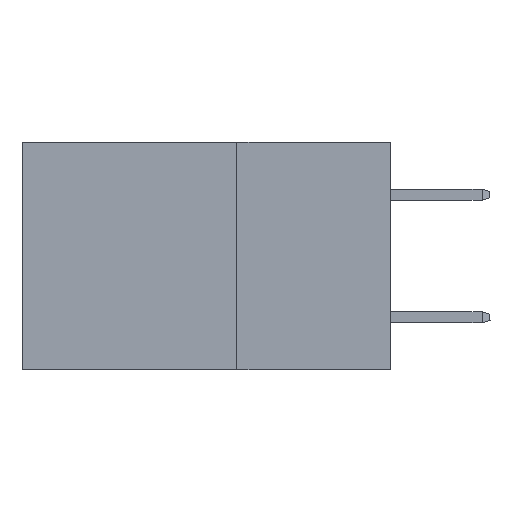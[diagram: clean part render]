
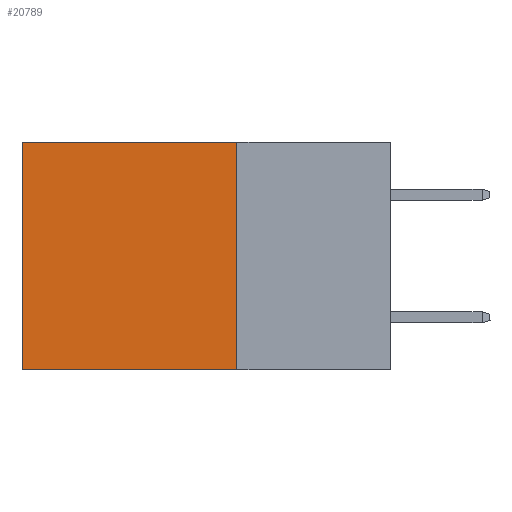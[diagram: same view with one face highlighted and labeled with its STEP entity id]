
A CAD part, left-side view. The second image highlights one B-rep face of the part: STEP entity #20789.
In plain terms, the highlighted planar face has unit normal (-1, 0, 0).
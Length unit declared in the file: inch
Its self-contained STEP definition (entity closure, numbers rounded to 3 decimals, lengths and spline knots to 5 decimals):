
#179 = DIRECTION ( 'NONE',  ( 0., 0., -1. ) ) ;
#887 = CARTESIAN_POINT ( 'NONE',  ( 0.2875, 0.25, 0. ) ) ;
#1106 = ORIENTED_EDGE ( 'NONE', *, *, #20926, .F. ) ;
#1913 = CARTESIAN_POINT ( 'NONE',  ( 0.2875, 0.6, 0. ) ) ;
#2788 = VERTEX_POINT ( 'NONE', #16098 ) ;
#2804 = CARTESIAN_POINT ( 'NONE',  ( 0.2875, 0.6, -0.37 ) ) ;
#3386 = VECTOR ( 'NONE', #23028, 39.37008 ) ;
#3429 = DIRECTION ( 'NONE',  ( 1., 0., 0. ) ) ;
#5271 = LINE ( 'NONE', #19650, #3386 ) ;
#5788 = CARTESIAN_POINT ( 'NONE',  ( 0.2875, 0.6, 0. ) ) ;
#6047 = DIRECTION ( 'NONE',  ( 0., 0., -1. ) ) ;
#6865 = LINE ( 'NONE', #1913, #8237 ) ;
#7371 = CARTESIAN_POINT ( 'NONE',  ( 0.2875, 0.25, 0. ) ) ;
#8237 = VECTOR ( 'NONE', #12826, 39.37008 ) ;
#9222 = ORIENTED_EDGE ( 'NONE', *, *, #9916, .T. ) ;
#9916 = EDGE_CURVE ( 'NONE', #11110, #18434, #6865, .T. ) ;
#11110 = VERTEX_POINT ( 'NONE', #5788 ) ;
#11276 = AXIS2_PLACEMENT_3D ( 'NONE', #7371, #3429, #179 ) ;
#12034 = ORIENTED_EDGE ( 'NONE', *, *, #20275, .T. ) ;
#12826 = DIRECTION ( 'NONE',  ( 0., 0., -1. ) ) ;
#13476 = CARTESIAN_POINT ( 'NONE',  ( 0.2875, 0.25, 0. ) ) ;
#14919 = EDGE_CURVE ( 'NONE', #2788, #18434, #17965, .T. ) ;
#16098 = CARTESIAN_POINT ( 'NONE',  ( 0.2875, 0.25, -0.37 ) ) ;
#16607 = FACE_OUTER_BOUND ( 'NONE', #20144, .T. ) ;
#17002 = VECTOR ( 'NONE', #6047, 39.37008 ) ;
#17801 = VECTOR ( 'NONE', #21571, 39.37008 ) ;
#17965 = LINE ( 'NONE', #19639, #17801 ) ;
#18434 = VERTEX_POINT ( 'NONE', #2804 ) ;
#19639 = CARTESIAN_POINT ( 'NONE',  ( 0.2875, 0.25, -0.37 ) ) ;
#19650 = CARTESIAN_POINT ( 'NONE',  ( 0.2875, 0.25, 0. ) ) ;
#20144 = EDGE_LOOP ( 'NONE', ( #9222, #21364, #1106, #12034 ) ) ;
#20275 = EDGE_CURVE ( 'NONE', #22296, #11110, #5271, .T. ) ;
#20789 = ADVANCED_FACE ( 'NONE', ( #16607 ), #23213, .F. ) ;
#20926 = EDGE_CURVE ( 'NONE', #22296, #2788, #22728, .T. ) ;
#21364 = ORIENTED_EDGE ( 'NONE', *, *, #14919, .F. ) ;
#21571 = DIRECTION ( 'NONE',  ( 0., 1., 0. ) ) ;
#22296 = VERTEX_POINT ( 'NONE', #887 ) ;
#22728 = LINE ( 'NONE', #13476, #17002 ) ;
#23028 = DIRECTION ( 'NONE',  ( 0., 1., 0. ) ) ;
#23213 = PLANE ( 'NONE',  #11276 ) ;
